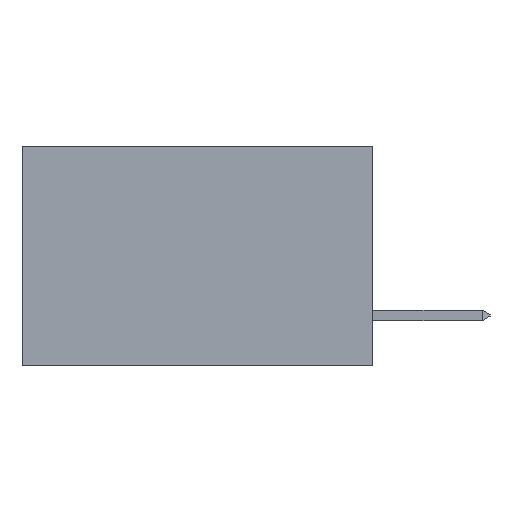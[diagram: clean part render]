
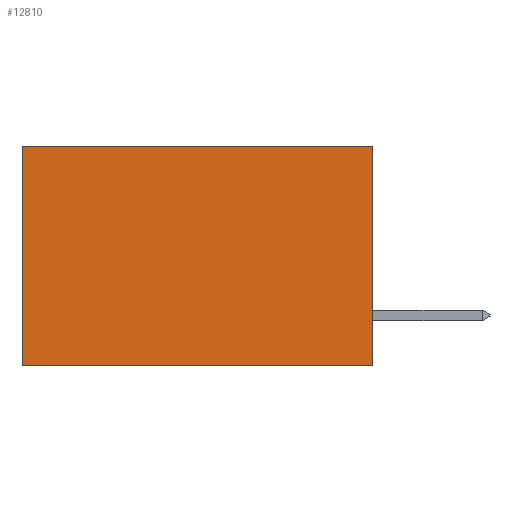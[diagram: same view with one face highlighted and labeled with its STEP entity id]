
A CAD part, left-side view. The second image highlights one B-rep face of the part: STEP entity #12810.
In plain terms, the highlighted planar face has unit normal (-1, 0, 0).
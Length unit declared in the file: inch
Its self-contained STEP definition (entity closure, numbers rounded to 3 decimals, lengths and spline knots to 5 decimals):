
#1705 = LINE ( 'NONE', #9516, #10746 ) ;
#1717 = CARTESIAN_POINT ( 'NONE',  ( 0.277, 0., -0.37 ) ) ;
#1875 = ORIENTED_EDGE ( 'NONE', *, *, #4605, .F. ) ;
#1968 = ORIENTED_EDGE ( 'NONE', *, *, #11902, .F. ) ;
#2066 = ORIENTED_EDGE ( 'NONE', *, *, #7733, .T. ) ;
#2764 = VECTOR ( 'NONE', #13057, 39.37008 ) ;
#2975 = PLANE ( 'NONE',  #6916 ) ;
#4136 = CARTESIAN_POINT ( 'NONE',  ( 0.277, 0., -0.37 ) ) ;
#4194 = CARTESIAN_POINT ( 'NONE',  ( 0.277, 0.59, -0.37 ) ) ;
#4605 = EDGE_CURVE ( 'NONE', #12719, #8724, #11813, .T. ) ;
#5241 = DIRECTION ( 'NONE',  ( 0., 0., -1. ) ) ;
#5423 = CARTESIAN_POINT ( 'NONE',  ( 0.277, 0.59, 0. ) ) ;
#5742 = EDGE_LOOP ( 'NONE', ( #11595, #1875, #1968, #2066 ) ) ;
#6048 = VECTOR ( 'NONE', #10147, 39.37008 ) ;
#6587 = VECTOR ( 'NONE', #13266, 39.37008 ) ;
#6916 = AXIS2_PLACEMENT_3D ( 'NONE', #4136, #11703, #5241 ) ;
#7733 = EDGE_CURVE ( 'NONE', #12735, #10627, #12748, .T. ) ;
#8724 = VERTEX_POINT ( 'NONE', #4194 ) ;
#9516 = CARTESIAN_POINT ( 'NONE',  ( 0.277, 0.59, -0.37 ) ) ;
#10147 = DIRECTION ( 'NONE',  ( 0., 1., 0. ) ) ;
#10266 = DIRECTION ( 'NONE',  ( 0., 0., -1. ) ) ;
#10465 = CARTESIAN_POINT ( 'NONE',  ( 0.277, 0., 0. ) ) ;
#10627 = VERTEX_POINT ( 'NONE', #5423 ) ;
#10709 = EDGE_CURVE ( 'NONE', #10627, #8724, #1705, .T. ) ;
#10746 = VECTOR ( 'NONE', #10266, 39.37008 ) ;
#10763 = CARTESIAN_POINT ( 'NONE',  ( 0.277, 0., -0.37 ) ) ;
#11403 = LINE ( 'NONE', #13260, #2764 ) ;
#11595 = ORIENTED_EDGE ( 'NONE', *, *, #10709, .T. ) ;
#11703 = DIRECTION ( 'NONE',  ( 1., 0., 0. ) ) ;
#11813 = LINE ( 'NONE', #10763, #6048 ) ;
#11902 = EDGE_CURVE ( 'NONE', #12735, #12719, #11403, .T. ) ;
#12719 = VERTEX_POINT ( 'NONE', #1717 ) ;
#12735 = VERTEX_POINT ( 'NONE', #10465 ) ;
#12748 = LINE ( 'NONE', #13228, #6587 ) ;
#12810 = ADVANCED_FACE ( 'NONE', ( #13807 ), #2975, .F. ) ;
#13057 = DIRECTION ( 'NONE',  ( 0., 0., -1. ) ) ;
#13228 = CARTESIAN_POINT ( 'NONE',  ( 0.277, 0., 0. ) ) ;
#13260 = CARTESIAN_POINT ( 'NONE',  ( 0.277, 0., -0.37 ) ) ;
#13266 = DIRECTION ( 'NONE',  ( 0., 1., 0. ) ) ;
#13807 = FACE_OUTER_BOUND ( 'NONE', #5742, .T. ) ;
